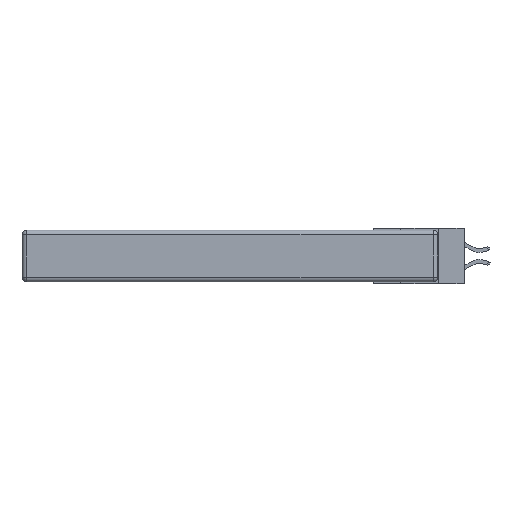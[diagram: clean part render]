
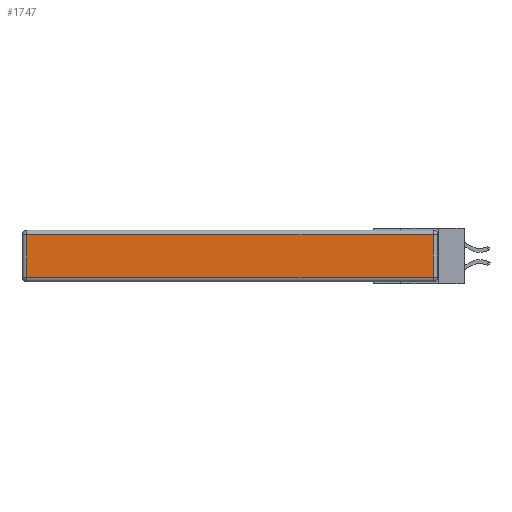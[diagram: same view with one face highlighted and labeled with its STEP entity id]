
A CAD part, left-side view. The second image highlights one B-rep face of the part: STEP entity #1747.
In plain terms, the highlighted planar face has unit normal (-1, 0, 0).
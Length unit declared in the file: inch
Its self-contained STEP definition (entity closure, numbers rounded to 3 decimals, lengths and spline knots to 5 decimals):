
#186 = ORIENTED_EDGE ( 'NONE', *, *, #13814, .T. ) ;
#306 = DIRECTION ( 'NONE',  ( 0., 0., -1. ) ) ;
#433 = VECTOR ( 'NONE', #13336, 39.37008 ) ;
#955 = VECTOR ( 'NONE', #15633, 39.37008 ) ;
#1347 = CARTESIAN_POINT ( 'NONE',  ( 0., 2.72, -0.313 ) ) ;
#1747 = ADVANCED_FACE ( 'NONE', ( #5948 ), #2880, .T. ) ;
#2230 = ORIENTED_EDGE ( 'NONE', *, *, #5766, .T. ) ;
#2312 = VECTOR ( 'NONE', #7553, 39.37008 ) ;
#2880 = PLANE ( 'NONE',  #13841 ) ;
#3148 = VERTEX_POINT ( 'NONE', #15277 ) ;
#3683 = LINE ( 'NONE', #5996, #433 ) ;
#3812 = CARTESIAN_POINT ( 'NONE',  ( 0., 0., -0.313 ) ) ;
#3960 = CARTESIAN_POINT ( 'NONE',  ( 0., 2.72, -0.03 ) ) ;
#4068 = EDGE_CURVE ( 'NONE', #3148, #11903, #3683, .T. ) ;
#4084 = DIRECTION ( 'NONE',  ( -1., 0., 0. ) ) ;
#4141 = DIRECTION ( 'NONE',  ( 0., 0., 1. ) ) ;
#5266 = CARTESIAN_POINT ( 'NONE',  ( 0., 0.03, -0.03 ) ) ;
#5403 = EDGE_CURVE ( 'NONE', #15634, #3148, #5915, .T. ) ;
#5475 = EDGE_LOOP ( 'NONE', ( #13562, #6398, #2230, #186 ) ) ;
#5766 = EDGE_CURVE ( 'NONE', #11903, #7946, #10606, .T. ) ;
#5915 = LINE ( 'NONE', #3812, #2312 ) ;
#5948 = FACE_OUTER_BOUND ( 'NONE', #5475, .T. ) ;
#5996 = CARTESIAN_POINT ( 'NONE',  ( 0., 0.03, -0.343 ) ) ;
#6398 = ORIENTED_EDGE ( 'NONE', *, *, #4068, .T. ) ;
#7553 = DIRECTION ( 'NONE',  ( 0., -1., 0. ) ) ;
#7946 = VERTEX_POINT ( 'NONE', #3960 ) ;
#7967 = VECTOR ( 'NONE', #306, 39.37008 ) ;
#10606 = LINE ( 'NONE', #14433, #955 ) ;
#11331 = CARTESIAN_POINT ( 'NONE',  ( 0., 0., -0.343 ) ) ;
#11903 = VERTEX_POINT ( 'NONE', #5266 ) ;
#12926 = LINE ( 'NONE', #14630, #7967 ) ;
#13336 = DIRECTION ( 'NONE',  ( 0., 0., 1. ) ) ;
#13562 = ORIENTED_EDGE ( 'NONE', *, *, #5403, .T. ) ;
#13814 = EDGE_CURVE ( 'NONE', #7946, #15634, #12926, .T. ) ;
#13841 = AXIS2_PLACEMENT_3D ( 'NONE', #11331, #4084, #4141 ) ;
#14433 = CARTESIAN_POINT ( 'NONE',  ( 0., 2.75, -0.03 ) ) ;
#14630 = CARTESIAN_POINT ( 'NONE',  ( 0., 2.72, -0.343 ) ) ;
#15277 = CARTESIAN_POINT ( 'NONE',  ( 0., 0.03, -0.313 ) ) ;
#15633 = DIRECTION ( 'NONE',  ( 0., 1., 0. ) ) ;
#15634 = VERTEX_POINT ( 'NONE', #1347 ) ;
